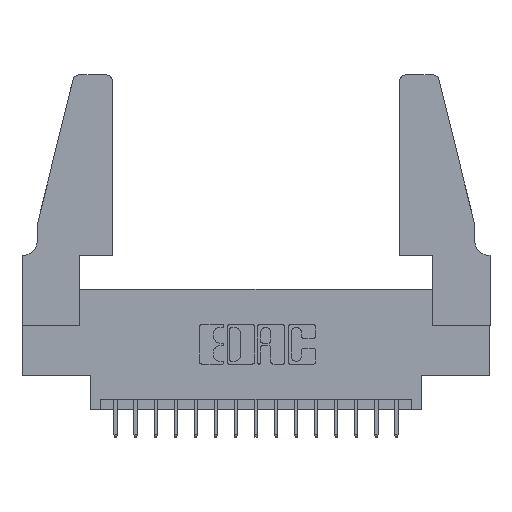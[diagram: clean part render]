
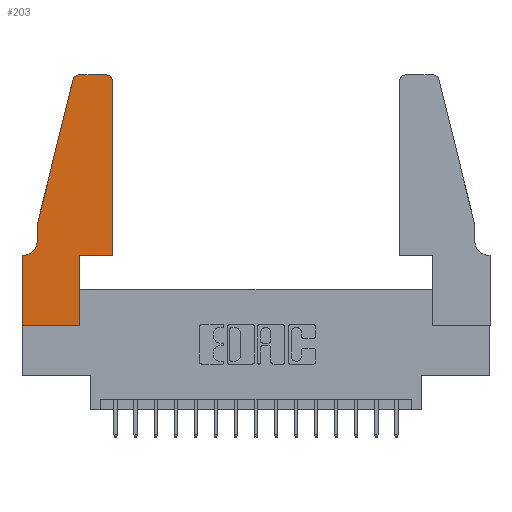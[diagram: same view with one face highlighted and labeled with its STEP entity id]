
A CAD part, top view. The second image highlights one B-rep face of the part: STEP entity #203.
In plain terms, the highlighted planar face has unit normal (0, 0, 1).
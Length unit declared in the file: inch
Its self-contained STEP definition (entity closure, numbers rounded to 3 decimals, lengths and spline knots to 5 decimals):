
#203 = ADVANCED_FACE ( 'NONE', ( #1376 ), #10777, .T. ) ;
#232 = CARTESIAN_POINT ( 'NONE',  ( 0.4205, 1.22, 0.37 ) ) ;
#582 = VERTEX_POINT ( 'NONE', #2237 ) ;
#703 = VERTEX_POINT ( 'NONE', #2401 ) ;
#756 = LINE ( 'NONE', #13058, #15749 ) ;
#1037 = CARTESIAN_POINT ( 'NONE',  ( 0.4505, 0.35, 0.37 ) ) ;
#1100 = CARTESIAN_POINT ( 'NONE',  ( 0., 0., 0.37 ) ) ;
#1170 = DIRECTION ( 'NONE',  ( -1., 0., 0. ) ) ;
#1376 = FACE_OUTER_BOUND ( 'NONE', #13878, .T. ) ;
#1446 = DIRECTION ( 'NONE',  ( 1., 0., 0. ) ) ;
#1603 = EDGE_CURVE ( 'NONE', #7105, #10051, #11506, .T. ) ;
#2237 = CARTESIAN_POINT ( 'NONE',  ( 0.2865, 0.35, 0.37 ) ) ;
#2401 = CARTESIAN_POINT ( 'NONE',  ( 0.284, 1.25, 0.37 ) ) ;
#2438 = LINE ( 'NONE', #5383, #15003 ) ;
#2459 = DIRECTION ( 'NONE',  ( 1., 0., 0. ) ) ;
#2721 = ORIENTED_EDGE ( 'NONE', *, *, #1603, .T. ) ;
#2791 = EDGE_CURVE ( 'NONE', #13328, #9945, #9339, .T. ) ;
#3006 = CIRCLE ( 'NONE', #10435, 0.03 ) ;
#3514 = ORIENTED_EDGE ( 'NONE', *, *, #2791, .T. ) ;
#3539 = DIRECTION ( 'NONE',  ( 0., 0., -1. ) ) ;
#3712 = DIRECTION ( 'NONE',  ( 0., -1., 0. ) ) ;
#3779 = DIRECTION ( 'NONE',  ( 1., 0., 0. ) ) ;
#3831 = DIRECTION ( 'NONE',  ( -0.239, -0.971, 0. ) ) ;
#3941 = VERTEX_POINT ( 'NONE', #8484 ) ;
#3970 = LINE ( 'NONE', #1100, #11829 ) ;
#4359 = AXIS2_PLACEMENT_3D ( 'NONE', #232, #5716, #9454 ) ;
#4697 = ORIENTED_EDGE ( 'NONE', *, *, #11790, .T. ) ;
#4802 = DIRECTION ( 'NONE',  ( -1., 0., 0. ) ) ;
#4892 = EDGE_CURVE ( 'NONE', #3941, #13901, #6148, .T. ) ;
#5383 = CARTESIAN_POINT ( 'NONE',  ( 0.2605, 1.25, 0.37 ) ) ;
#5716 = DIRECTION ( 'NONE',  ( 0., 0., 1. ) ) ;
#6123 = CARTESIAN_POINT ( 'NONE',  ( 0., 0.35, 0.37 ) ) ;
#6148 = LINE ( 'NONE', #11604, #6467 ) ;
#6210 = VERTEX_POINT ( 'NONE', #13182 ) ;
#6293 = CARTESIAN_POINT ( 'NONE',  ( 0.0055, 0.42, 0.37 ) ) ;
#6467 = VECTOR ( 'NONE', #4802, 39.37008 ) ;
#6473 = CARTESIAN_POINT ( 'NONE',  ( 0.2865, 0.35, 0.37 ) ) ;
#6491 = ORIENTED_EDGE ( 'NONE', *, *, #16402, .T. ) ;
#6496 = DIRECTION ( 'NONE',  ( 1., 0., 0. ) ) ;
#6557 = CARTESIAN_POINT ( 'NONE',  ( 0.284, 1.22, 0.37 ) ) ;
#7105 = VERTEX_POINT ( 'NONE', #8834 ) ;
#7367 = ORIENTED_EDGE ( 'NONE', *, *, #8594, .T. ) ;
#7377 = ORIENTED_EDGE ( 'NONE', *, *, #16962, .T. ) ;
#7608 = CARTESIAN_POINT ( 'NONE',  ( 0.25487, 1.22718, 0.37 ) ) ;
#7781 = DIRECTION ( 'NONE',  ( 0., -1., 0. ) ) ;
#7985 = ORIENTED_EDGE ( 'NONE', *, *, #11105, .T. ) ;
#8082 = CARTESIAN_POINT ( 'NONE',  ( 0.0755, 0.5, 0.37 ) ) ;
#8255 = VECTOR ( 'NONE', #16083, 39.37008 ) ;
#8342 = CARTESIAN_POINT ( 'NONE',  ( 0., 0., 0.37 ) ) ;
#8484 = CARTESIAN_POINT ( 'NONE',  ( 0.0055, 0.35, 0.37 ) ) ;
#8594 = EDGE_CURVE ( 'NONE', #13901, #15021, #10748, .T. ) ;
#8668 = EDGE_CURVE ( 'NONE', #6210, #582, #9475, .T. ) ;
#8814 = CIRCLE ( 'NONE', #16020, 0.07 ) ;
#8834 = CARTESIAN_POINT ( 'NONE',  ( 0.4505, 1.22, 0.37 ) ) ;
#8971 = DIRECTION ( 'NONE',  ( -1., 0., 0. ) ) ;
#9339 = LINE ( 'NONE', #8082, #9817 ) ;
#9454 = DIRECTION ( 'NONE',  ( 1., 0., 0. ) ) ;
#9475 = LINE ( 'NONE', #6473, #8255 ) ;
#9817 = VECTOR ( 'NONE', #3712, 39.37008 ) ;
#9945 = VERTEX_POINT ( 'NONE', #14278 ) ;
#10051 = VERTEX_POINT ( 'NONE', #13385 ) ;
#10184 = EDGE_CURVE ( 'NONE', #12115, #13328, #14698, .T. ) ;
#10435 = AXIS2_PLACEMENT_3D ( 'NONE', #6557, #10579, #3779 ) ;
#10579 = DIRECTION ( 'NONE',  ( 0., 0., 1. ) ) ;
#10622 = CARTESIAN_POINT ( 'NONE',  ( 0.0755, 0.5, 0.37 ) ) ;
#10748 = LINE ( 'NONE', #12210, #11994 ) ;
#10777 = PLANE ( 'NONE',  #11479 ) ;
#10937 = EDGE_CURVE ( 'NONE', #9945, #3941, #8814, .T. ) ;
#11105 = EDGE_CURVE ( 'NONE', #703, #12115, #3006, .T. ) ;
#11479 = AXIS2_PLACEMENT_3D ( 'NONE', #17495, #17793, #2459 ) ;
#11506 = CIRCLE ( 'NONE', #4359, 0.03 ) ;
#11604 = CARTESIAN_POINT ( 'NONE',  ( 0.0755, 0.35, 0.37 ) ) ;
#11790 = EDGE_CURVE ( 'NONE', #12515, #7105, #756, .T. ) ;
#11821 = VECTOR ( 'NONE', #3831, 39.37008 ) ;
#11829 = VECTOR ( 'NONE', #6496, 39.37008 ) ;
#11855 = LINE ( 'NONE', #12130, #15297 ) ;
#11994 = VECTOR ( 'NONE', #7781, 39.37008 ) ;
#12115 = VERTEX_POINT ( 'NONE', #7608 ) ;
#12130 = CARTESIAN_POINT ( 'NONE',  ( 0.4505, 0.35, 0.37 ) ) ;
#12210 = CARTESIAN_POINT ( 'NONE',  ( 0., 0., 0.37 ) ) ;
#12515 = VERTEX_POINT ( 'NONE', #1037 ) ;
#12787 = ORIENTED_EDGE ( 'NONE', *, *, #10937, .T. ) ;
#13058 = CARTESIAN_POINT ( 'NONE',  ( 0.4505, 0.35, 0.37 ) ) ;
#13134 = ORIENTED_EDGE ( 'NONE', *, *, #4892, .T. ) ;
#13142 = CARTESIAN_POINT ( 'NONE',  ( 0.0755, 0.5, 0.37 ) ) ;
#13157 = ORIENTED_EDGE ( 'NONE', *, *, #17640, .T. ) ;
#13161 = ORIENTED_EDGE ( 'NONE', *, *, #10184, .T. ) ;
#13182 = CARTESIAN_POINT ( 'NONE',  ( 0.2865, 0., 0.37 ) ) ;
#13328 = VERTEX_POINT ( 'NONE', #13142 ) ;
#13385 = CARTESIAN_POINT ( 'NONE',  ( 0.4205, 1.25, 0.37 ) ) ;
#13878 = EDGE_LOOP ( 'NONE', ( #7377, #7985, #13161, #3514, #12787, #13134, #7367, #13157, #15367, #6491, #4697, #2721 ) ) ;
#13901 = VERTEX_POINT ( 'NONE', #6123 ) ;
#14278 = CARTESIAN_POINT ( 'NONE',  ( 0.0755, 0.42, 0.37 ) ) ;
#14698 = LINE ( 'NONE', #10622, #11821 ) ;
#15003 = VECTOR ( 'NONE', #1170, 39.37008 ) ;
#15021 = VERTEX_POINT ( 'NONE', #8342 ) ;
#15297 = VECTOR ( 'NONE', #1446, 39.37008 ) ;
#15367 = ORIENTED_EDGE ( 'NONE', *, *, #8668, .T. ) ;
#15749 = VECTOR ( 'NONE', #15919, 39.37008 ) ;
#15919 = DIRECTION ( 'NONE',  ( 0., 1., 0. ) ) ;
#16020 = AXIS2_PLACEMENT_3D ( 'NONE', #6293, #3539, #8971 ) ;
#16083 = DIRECTION ( 'NONE',  ( 0., 1., 0. ) ) ;
#16402 = EDGE_CURVE ( 'NONE', #582, #12515, #11855, .T. ) ;
#16962 = EDGE_CURVE ( 'NONE', #10051, #703, #2438, .T. ) ;
#17495 = CARTESIAN_POINT ( 'NONE',  ( 0., 0.35, 0.37 ) ) ;
#17640 = EDGE_CURVE ( 'NONE', #15021, #6210, #3970, .T. ) ;
#17793 = DIRECTION ( 'NONE',  ( 0., 0., 1. ) ) ;
